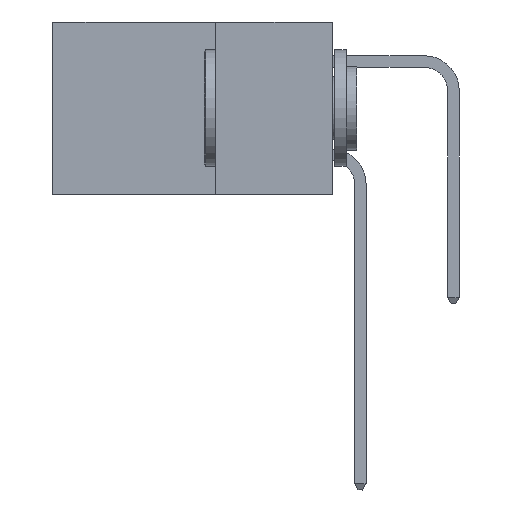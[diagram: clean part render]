
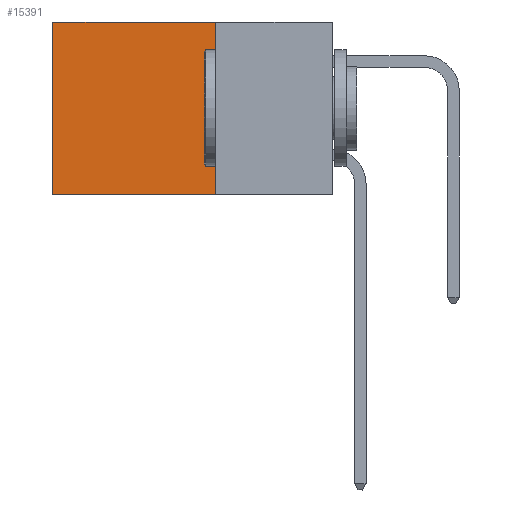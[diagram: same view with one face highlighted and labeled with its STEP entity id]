
A CAD part, left-side view. The second image highlights one B-rep face of the part: STEP entity #15391.
In plain terms, the highlighted planar face has unit normal (-1, 0, 0).
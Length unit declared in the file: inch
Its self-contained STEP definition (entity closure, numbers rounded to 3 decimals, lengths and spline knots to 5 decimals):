
#184 = DIRECTION ( 'NONE',  ( 0., 0., -1. ) ) ;
#439 = CARTESIAN_POINT ( 'NONE',  ( 0.298, 0.6, -0.37 ) ) ;
#1347 = EDGE_LOOP ( 'NONE', ( #15133, #3945, #13956, #11209 ) ) ;
#2902 = VECTOR ( 'NONE', #3467, 39.37008 ) ;
#3352 = CARTESIAN_POINT ( 'NONE',  ( 0.298, 0.25, 0. ) ) ;
#3467 = DIRECTION ( 'NONE',  ( 0., 0., -1. ) ) ;
#3945 = ORIENTED_EDGE ( 'NONE', *, *, #13289, .F. ) ;
#4189 = EDGE_CURVE ( 'NONE', #9147, #16525, #6892, .T. ) ;
#6227 = VECTOR ( 'NONE', #16111, 39.37008 ) ;
#6844 = DIRECTION ( 'NONE',  ( 1., 0., 0. ) ) ;
#6892 = LINE ( 'NONE', #10729, #16504 ) ;
#9127 = VECTOR ( 'NONE', #10693, 39.37008 ) ;
#9147 = VERTEX_POINT ( 'NONE', #14665 ) ;
#9290 = CARTESIAN_POINT ( 'NONE',  ( 0.298, 0.25, 0. ) ) ;
#9409 = AXIS2_PLACEMENT_3D ( 'NONE', #16165, #6844, #10973 ) ;
#10654 = LINE ( 'NONE', #3352, #2902 ) ;
#10693 = DIRECTION ( 'NONE',  ( 0., 1., 0. ) ) ;
#10699 = EDGE_CURVE ( 'NONE', #11858, #15419, #10654, .T. ) ;
#10729 = CARTESIAN_POINT ( 'NONE',  ( 0.298, 0.6, 0. ) ) ;
#10973 = DIRECTION ( 'NONE',  ( 0., 0., -1. ) ) ;
#11209 = ORIENTED_EDGE ( 'NONE', *, *, #16440, .T. ) ;
#11858 = VERTEX_POINT ( 'NONE', #16593 ) ;
#12128 = CARTESIAN_POINT ( 'NONE',  ( 0.298, 0.25, -0.37 ) ) ;
#13289 = EDGE_CURVE ( 'NONE', #15419, #16525, #16088, .T. ) ;
#13308 = CARTESIAN_POINT ( 'NONE',  ( 0.298, 0.25, -0.37 ) ) ;
#13357 = PLANE ( 'NONE',  #9409 ) ;
#13956 = ORIENTED_EDGE ( 'NONE', *, *, #10699, .F. ) ;
#14665 = CARTESIAN_POINT ( 'NONE',  ( 0.298, 0.6, 0. ) ) ;
#15133 = ORIENTED_EDGE ( 'NONE', *, *, #4189, .T. ) ;
#15391 = ADVANCED_FACE ( 'NONE', ( #16470 ), #13357, .F. ) ;
#15419 = VERTEX_POINT ( 'NONE', #13308 ) ;
#16088 = LINE ( 'NONE', #12128, #9127 ) ;
#16111 = DIRECTION ( 'NONE',  ( 0., 1., 0. ) ) ;
#16165 = CARTESIAN_POINT ( 'NONE',  ( 0.298, 0.25, 0. ) ) ;
#16440 = EDGE_CURVE ( 'NONE', #11858, #9147, #16641, .T. ) ;
#16470 = FACE_OUTER_BOUND ( 'NONE', #1347, .T. ) ;
#16504 = VECTOR ( 'NONE', #184, 39.37008 ) ;
#16525 = VERTEX_POINT ( 'NONE', #439 ) ;
#16593 = CARTESIAN_POINT ( 'NONE',  ( 0.298, 0.25, 0. ) ) ;
#16641 = LINE ( 'NONE', #9290, #6227 ) ;
